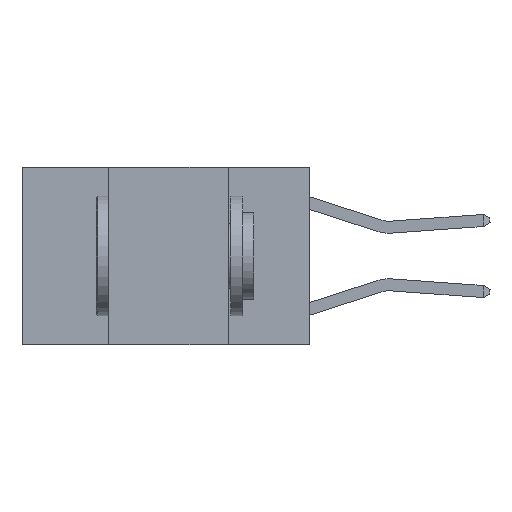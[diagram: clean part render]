
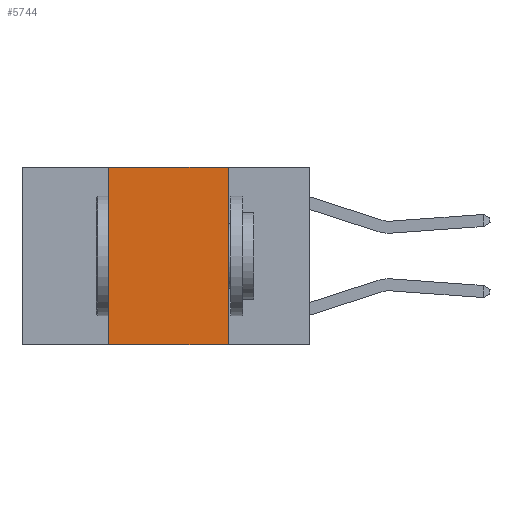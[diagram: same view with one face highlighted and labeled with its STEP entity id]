
A CAD part, left-side view. The second image highlights one B-rep face of the part: STEP entity #5744.
In plain terms, the highlighted planar face has unit normal (-1, 0, 0).
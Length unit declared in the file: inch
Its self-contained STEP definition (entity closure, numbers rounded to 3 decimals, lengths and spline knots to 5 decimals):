
#695 = VERTEX_POINT ( 'NONE', #8656 ) ;
#723 = VERTEX_POINT ( 'NONE', #12441 ) ;
#761 = VERTEX_POINT ( 'NONE', #3838 ) ;
#1523 = DIRECTION ( 'NONE',  ( 0., 0., -1. ) ) ;
#1774 = PLANE ( 'NONE',  #2642 ) ;
#2037 = DIRECTION ( 'NONE',  ( 1., 0., 0. ) ) ;
#2161 = DIRECTION ( 'NONE',  ( 0., -1., 0. ) ) ;
#2642 = AXIS2_PLACEMENT_3D ( 'NONE', #2885, #2037, #4297 ) ;
#2817 = CARTESIAN_POINT ( 'NONE',  ( 0., 0.42, 0. ) ) ;
#2885 = CARTESIAN_POINT ( 'NONE',  ( 0., 0.6, 0. ) ) ;
#3422 = CARTESIAN_POINT ( 'NONE',  ( 0., 0.17, 0. ) ) ;
#3435 = ORIENTED_EDGE ( 'NONE', *, *, #10925, .F. ) ;
#3838 = CARTESIAN_POINT ( 'NONE',  ( 0., 0.42, 0. ) ) ;
#3936 = EDGE_LOOP ( 'NONE', ( #3435, #4194, #11505, #7965 ) ) ;
#4194 = ORIENTED_EDGE ( 'NONE', *, *, #8308, .F. ) ;
#4297 = DIRECTION ( 'NONE',  ( 0., 0., -1. ) ) ;
#5550 = VECTOR ( 'NONE', #2161, 39.37008 ) ;
#5744 = ADVANCED_FACE ( 'NONE', ( #10592 ), #1774, .F. ) ;
#5809 = CARTESIAN_POINT ( 'NONE',  ( 0., 0.17, 0. ) ) ;
#5855 = DIRECTION ( 'NONE',  ( 0., 0., 1. ) ) ;
#6495 = LINE ( 'NONE', #12353, #9976 ) ;
#6795 = VERTEX_POINT ( 'NONE', #5809 ) ;
#7615 = DIRECTION ( 'NONE',  ( 0., -1., 0. ) ) ;
#7899 = VECTOR ( 'NONE', #5855, 39.37008 ) ;
#7965 = ORIENTED_EDGE ( 'NONE', *, *, #12382, .T. ) ;
#8308 = EDGE_CURVE ( 'NONE', #761, #6795, #10138, .T. ) ;
#8656 = CARTESIAN_POINT ( 'NONE',  ( 0., 0.42, -0.37 ) ) ;
#9135 = VECTOR ( 'NONE', #1523, 39.37008 ) ;
#9976 = VECTOR ( 'NONE', #7615, 39.37008 ) ;
#10021 = CARTESIAN_POINT ( 'NONE',  ( 0., 0.6, 0. ) ) ;
#10138 = LINE ( 'NONE', #10021, #5550 ) ;
#10506 = LINE ( 'NONE', #2817, #7899 ) ;
#10592 = FACE_OUTER_BOUND ( 'NONE', #3936, .T. ) ;
#10925 = EDGE_CURVE ( 'NONE', #6795, #723, #12285, .T. ) ;
#10973 = EDGE_CURVE ( 'NONE', #695, #761, #10506, .T. ) ;
#11505 = ORIENTED_EDGE ( 'NONE', *, *, #10973, .F. ) ;
#12285 = LINE ( 'NONE', #3422, #9135 ) ;
#12353 = CARTESIAN_POINT ( 'NONE',  ( 0., 0.6, -0.37 ) ) ;
#12382 = EDGE_CURVE ( 'NONE', #695, #723, #6495, .T. ) ;
#12441 = CARTESIAN_POINT ( 'NONE',  ( 0., 0.17, -0.37 ) ) ;
